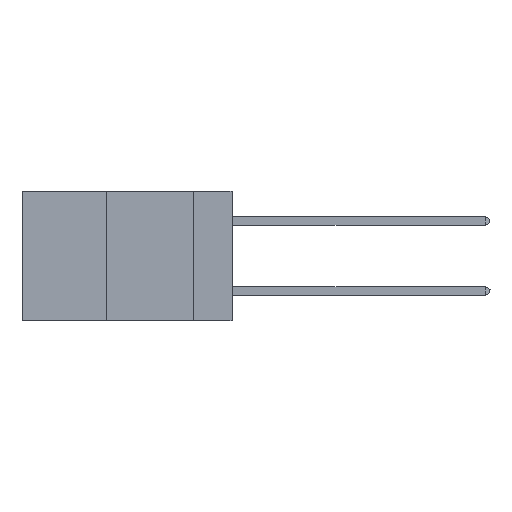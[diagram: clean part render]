
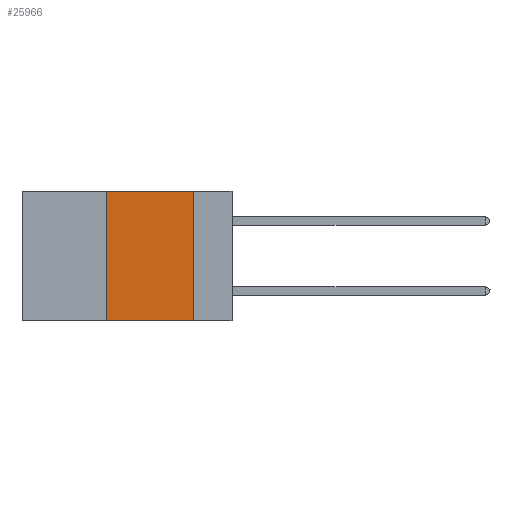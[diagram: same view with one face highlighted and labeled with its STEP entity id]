
A CAD part, left-side view. The second image highlights one B-rep face of the part: STEP entity #25966.
In plain terms, the highlighted planar face has unit normal (-1, 0, 0).
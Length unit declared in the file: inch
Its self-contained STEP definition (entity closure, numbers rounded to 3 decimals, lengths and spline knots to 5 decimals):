
#259 = ORIENTED_EDGE ( 'NONE', *, *, #24658, .T. ) ;
#289 = FACE_OUTER_BOUND ( 'NONE', #20689, .T. ) ;
#1353 = CARTESIAN_POINT ( 'NONE',  ( 0., 0.6, 0. ) ) ;
#2445 = AXIS2_PLACEMENT_3D ( 'NONE', #35608, #6589, #29279 ) ;
#5341 = LINE ( 'NONE', #26958, #6373 ) ;
#6136 = VECTOR ( 'NONE', #19785, 39.37008 ) ;
#6364 = CARTESIAN_POINT ( 'NONE',  ( 0., 0.11, -0.37 ) ) ;
#6373 = VECTOR ( 'NONE', #7517, 39.37008 ) ;
#6589 = DIRECTION ( 'NONE',  ( 1., 0., 0. ) ) ;
#7517 = DIRECTION ( 'NONE',  ( 0., 0., 1. ) ) ;
#9970 = CARTESIAN_POINT ( 'NONE',  ( 0., 0.6, -0.37 ) ) ;
#10574 = VECTOR ( 'NONE', #27421, 39.37008 ) ;
#11388 = VERTEX_POINT ( 'NONE', #12756 ) ;
#12756 = CARTESIAN_POINT ( 'NONE',  ( 0., 0.11, 0. ) ) ;
#13539 = ORIENTED_EDGE ( 'NONE', *, *, #39731, .F. ) ;
#14635 = CARTESIAN_POINT ( 'NONE',  ( 0., 0.11, 0. ) ) ;
#15032 = VERTEX_POINT ( 'NONE', #32632 ) ;
#16281 = PLANE ( 'NONE',  #2445 ) ;
#17846 = EDGE_CURVE ( 'NONE', #19938, #15032, #5341, .T. ) ;
#19785 = DIRECTION ( 'NONE',  ( 0., -1., 0. ) ) ;
#19938 = VERTEX_POINT ( 'NONE', #25583 ) ;
#20689 = EDGE_LOOP ( 'NONE', ( #13539, #24747, #21178, #259 ) ) ;
#21178 = ORIENTED_EDGE ( 'NONE', *, *, #17846, .F. ) ;
#24658 = EDGE_CURVE ( 'NONE', #19938, #29402, #32032, .T. ) ;
#24747 = ORIENTED_EDGE ( 'NONE', *, *, #35790, .F. ) ;
#25583 = CARTESIAN_POINT ( 'NONE',  ( 0., 0.36, -0.37 ) ) ;
#25966 = ADVANCED_FACE ( 'NONE', ( #289 ), #16281, .F. ) ;
#26958 = CARTESIAN_POINT ( 'NONE',  ( 0., 0.36, 0. ) ) ;
#27421 = DIRECTION ( 'NONE',  ( 0., -1., 0. ) ) ;
#29076 = LINE ( 'NONE', #14635, #37626 ) ;
#29279 = DIRECTION ( 'NONE',  ( 0., 0., -1. ) ) ;
#29402 = VERTEX_POINT ( 'NONE', #6364 ) ;
#31877 = LINE ( 'NONE', #1353, #10574 ) ;
#32032 = LINE ( 'NONE', #9970, #6136 ) ;
#32632 = CARTESIAN_POINT ( 'NONE',  ( 0., 0.36, 0. ) ) ;
#35608 = CARTESIAN_POINT ( 'NONE',  ( 0., 0.6, 0. ) ) ;
#35790 = EDGE_CURVE ( 'NONE', #15032, #11388, #31877, .T. ) ;
#37218 = DIRECTION ( 'NONE',  ( 0., 0., -1. ) ) ;
#37626 = VECTOR ( 'NONE', #37218, 39.37008 ) ;
#39731 = EDGE_CURVE ( 'NONE', #11388, #29402, #29076, .T. ) ;
